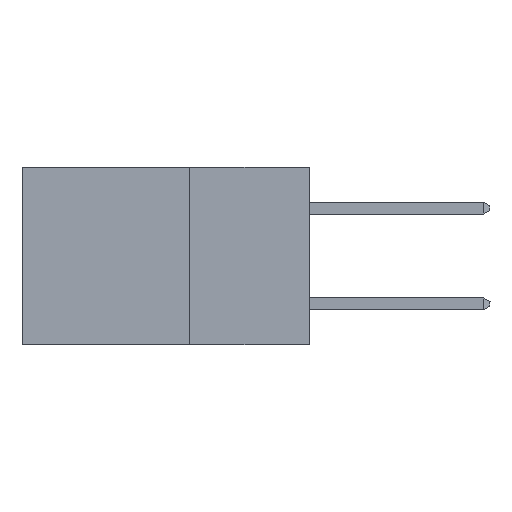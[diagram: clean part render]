
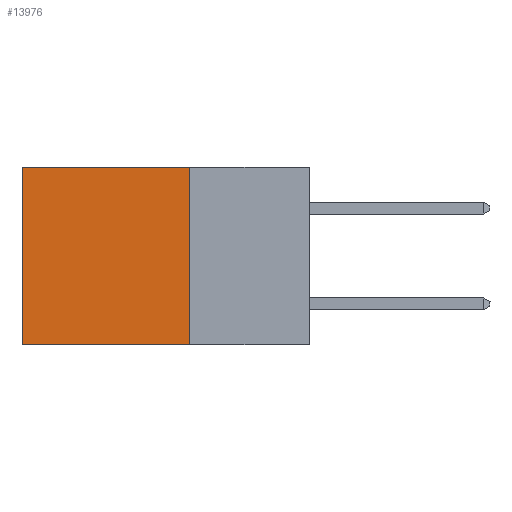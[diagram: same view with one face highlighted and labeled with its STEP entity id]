
A CAD part, left-side view. The second image highlights one B-rep face of the part: STEP entity #13976.
In plain terms, the highlighted planar face has unit normal (-1, 0, 0).
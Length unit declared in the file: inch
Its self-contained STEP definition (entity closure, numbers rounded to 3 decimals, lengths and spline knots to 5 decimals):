
#17 = FACE_OUTER_BOUND ( 'NONE', #15281, .T. ) ;
#291 = EDGE_CURVE ( 'NONE', #543, #7387, #4470, .T. ) ;
#543 = VERTEX_POINT ( 'NONE', #1450 ) ;
#1122 = DIRECTION ( 'NONE',  ( 0., 1., 0. ) ) ;
#1386 = AXIS2_PLACEMENT_3D ( 'NONE', #8916, #5697, #16134 ) ;
#1450 = CARTESIAN_POINT ( 'NONE',  ( 0.2875, 0.25, 0. ) ) ;
#2242 = ORIENTED_EDGE ( 'NONE', *, *, #291, .T. ) ;
#3911 = VECTOR ( 'NONE', #1122, 39.37008 ) ;
#4125 = CARTESIAN_POINT ( 'NONE',  ( 0.2875, 0.25, 0. ) ) ;
#4431 = VECTOR ( 'NONE', #18038, 39.37008 ) ;
#4470 = LINE ( 'NONE', #4125, #10546 ) ;
#4783 = EDGE_CURVE ( 'NONE', #543, #11427, #12798, .T. ) ;
#5147 = LINE ( 'NONE', #16232, #17743 ) ;
#5697 = DIRECTION ( 'NONE',  ( 1., 0., 0. ) ) ;
#6086 = VERTEX_POINT ( 'NONE', #12505 ) ;
#7044 = CARTESIAN_POINT ( 'NONE',  ( 0.2875, 0.6, 0. ) ) ;
#7387 = VERTEX_POINT ( 'NONE', #7044 ) ;
#8588 = LINE ( 'NONE', #11695, #3911 ) ;
#8916 = CARTESIAN_POINT ( 'NONE',  ( 0.2875, 0.25, 0. ) ) ;
#9133 = CARTESIAN_POINT ( 'NONE',  ( 0.2875, 0.25, -0.37 ) ) ;
#10301 = ORIENTED_EDGE ( 'NONE', *, *, #15477, .T. ) ;
#10366 = DIRECTION ( 'NONE',  ( 0., 0., -1. ) ) ;
#10546 = VECTOR ( 'NONE', #14857, 39.37008 ) ;
#11427 = VERTEX_POINT ( 'NONE', #9133 ) ;
#11695 = CARTESIAN_POINT ( 'NONE',  ( 0.2875, 0.25, -0.37 ) ) ;
#12505 = CARTESIAN_POINT ( 'NONE',  ( 0.2875, 0.6, -0.37 ) ) ;
#12798 = LINE ( 'NONE', #15321, #4431 ) ;
#13690 = ORIENTED_EDGE ( 'NONE', *, *, #17289, .F. ) ;
#13976 = ADVANCED_FACE ( 'NONE', ( #17 ), #14802, .F. ) ;
#14636 = ORIENTED_EDGE ( 'NONE', *, *, #4783, .F. ) ;
#14802 = PLANE ( 'NONE',  #1386 ) ;
#14857 = DIRECTION ( 'NONE',  ( 0., 1., 0. ) ) ;
#15281 = EDGE_LOOP ( 'NONE', ( #10301, #13690, #14636, #2242 ) ) ;
#15321 = CARTESIAN_POINT ( 'NONE',  ( 0.2875, 0.25, 0. ) ) ;
#15477 = EDGE_CURVE ( 'NONE', #7387, #6086, #5147, .T. ) ;
#16134 = DIRECTION ( 'NONE',  ( 0., 0., -1. ) ) ;
#16232 = CARTESIAN_POINT ( 'NONE',  ( 0.2875, 0.6, 0. ) ) ;
#17289 = EDGE_CURVE ( 'NONE', #11427, #6086, #8588, .T. ) ;
#17743 = VECTOR ( 'NONE', #10366, 39.37008 ) ;
#18038 = DIRECTION ( 'NONE',  ( 0., 0., -1. ) ) ;
